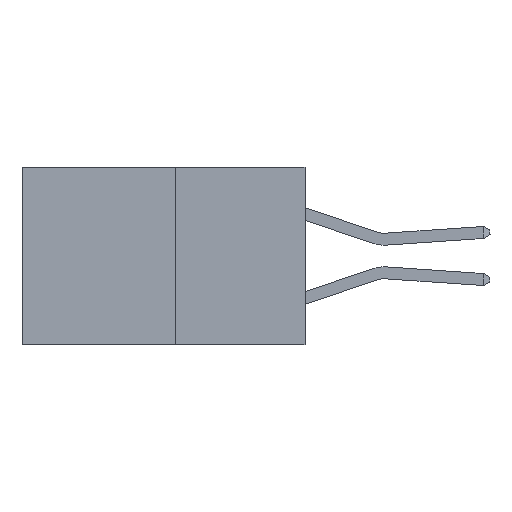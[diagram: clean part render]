
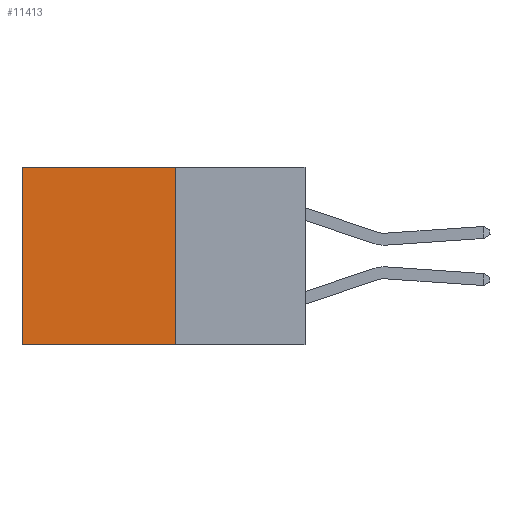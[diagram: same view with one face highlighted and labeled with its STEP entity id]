
A CAD part, left-side view. The second image highlights one B-rep face of the part: STEP entity #11413.
In plain terms, the highlighted planar face has unit normal (-1, 0, 0).
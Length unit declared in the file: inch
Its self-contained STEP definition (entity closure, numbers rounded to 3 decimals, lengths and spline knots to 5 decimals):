
#723 = CARTESIAN_POINT ( 'NONE',  ( 0.277, 0.59, 0. ) ) ;
#911 = ORIENTED_EDGE ( 'NONE', *, *, #5852, .F. ) ;
#1016 = EDGE_LOOP ( 'NONE', ( #19471, #911, #1211, #8833 ) ) ;
#1045 = AXIS2_PLACEMENT_3D ( 'NONE', #7194, #8969, #21302 ) ;
#1211 = ORIENTED_EDGE ( 'NONE', *, *, #5119, .F. ) ;
#1508 = CARTESIAN_POINT ( 'NONE',  ( 0.277, 0.27, -0.37 ) ) ;
#2557 = CARTESIAN_POINT ( 'NONE',  ( 0.277, 0.27, 0. ) ) ;
#3058 = DIRECTION ( 'NONE',  ( 0., 1., 0. ) ) ;
#3344 = LINE ( 'NONE', #14588, #16995 ) ;
#5119 = EDGE_CURVE ( 'NONE', #20204, #20596, #3344, .T. ) ;
#5411 = VECTOR ( 'NONE', #19971, 39.37008 ) ;
#5852 = EDGE_CURVE ( 'NONE', #20596, #12877, #14169, .T. ) ;
#7194 = CARTESIAN_POINT ( 'NONE',  ( 0.277, 0.27, -0.37 ) ) ;
#8629 = EDGE_CURVE ( 'NONE', #12310, #12877, #19519, .T. ) ;
#8833 = ORIENTED_EDGE ( 'NONE', *, *, #16717, .T. ) ;
#8969 = DIRECTION ( 'NONE',  ( 1., 0., 0. ) ) ;
#10253 = LINE ( 'NONE', #14205, #19109 ) ;
#10713 = DIRECTION ( 'NONE',  ( 0., 1., 0. ) ) ;
#11175 = CARTESIAN_POINT ( 'NONE',  ( 0.277, 0.59, -0.37 ) ) ;
#11413 = ADVANCED_FACE ( 'NONE', ( #18571 ), #17821, .F. ) ;
#12310 = VERTEX_POINT ( 'NONE', #723 ) ;
#12510 = CARTESIAN_POINT ( 'NONE',  ( 0.277, 0.27, -0.37 ) ) ;
#12877 = VERTEX_POINT ( 'NONE', #11175 ) ;
#13600 = VECTOR ( 'NONE', #3058, 39.37008 ) ;
#14169 = LINE ( 'NONE', #1508, #13600 ) ;
#14205 = CARTESIAN_POINT ( 'NONE',  ( 0.277, 0.27, 0. ) ) ;
#14588 = CARTESIAN_POINT ( 'NONE',  ( 0.277, 0.27, -0.37 ) ) ;
#15572 = DIRECTION ( 'NONE',  ( 0., 0., -1. ) ) ;
#16717 = EDGE_CURVE ( 'NONE', #20204, #12310, #10253, .T. ) ;
#16995 = VECTOR ( 'NONE', #15572, 39.37008 ) ;
#17821 = PLANE ( 'NONE',  #1045 ) ;
#18206 = CARTESIAN_POINT ( 'NONE',  ( 0.277, 0.59, -0.37 ) ) ;
#18571 = FACE_OUTER_BOUND ( 'NONE', #1016, .T. ) ;
#19109 = VECTOR ( 'NONE', #10713, 39.37008 ) ;
#19471 = ORIENTED_EDGE ( 'NONE', *, *, #8629, .T. ) ;
#19519 = LINE ( 'NONE', #18206, #5411 ) ;
#19971 = DIRECTION ( 'NONE',  ( 0., 0., -1. ) ) ;
#20204 = VERTEX_POINT ( 'NONE', #2557 ) ;
#20596 = VERTEX_POINT ( 'NONE', #12510 ) ;
#21302 = DIRECTION ( 'NONE',  ( 0., 0., -1. ) ) ;
